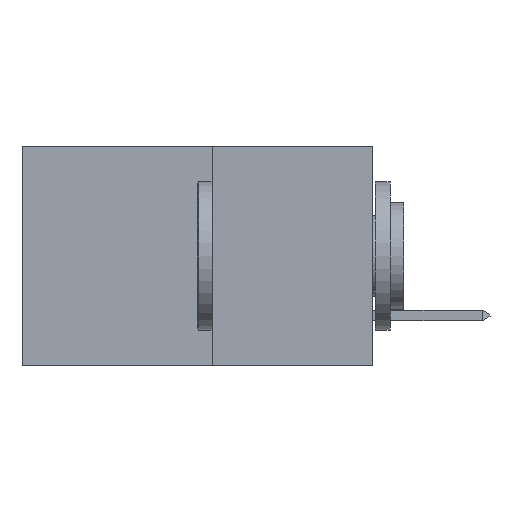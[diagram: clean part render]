
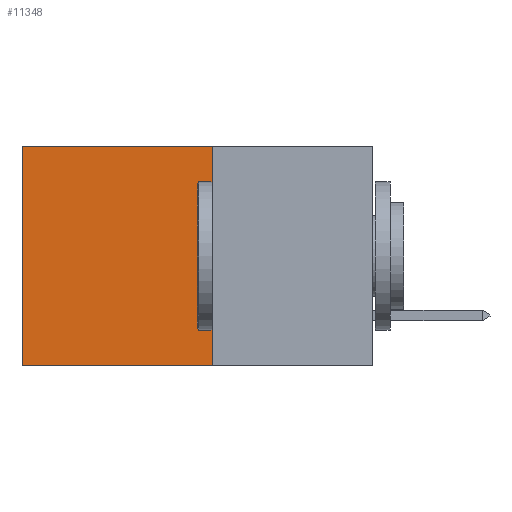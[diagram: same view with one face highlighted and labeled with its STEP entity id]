
A CAD part, left-side view. The second image highlights one B-rep face of the part: STEP entity #11348.
In plain terms, the highlighted planar face has unit normal (-1, 0, 0).
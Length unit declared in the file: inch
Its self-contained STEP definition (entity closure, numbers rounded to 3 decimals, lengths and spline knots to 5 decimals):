
#98 = FACE_OUTER_BOUND ( 'NONE', #2674, .T. ) ;
#156 = CARTESIAN_POINT ( 'NONE',  ( 0.277, 0.59, -0.37 ) ) ;
#1239 = ORIENTED_EDGE ( 'NONE', *, *, #2394, .F. ) ;
#1369 = VERTEX_POINT ( 'NONE', #7367 ) ;
#1559 = ORIENTED_EDGE ( 'NONE', *, *, #7161, .T. ) ;
#2394 = EDGE_CURVE ( 'NONE', #5105, #10106, #10455, .T. ) ;
#2674 = EDGE_LOOP ( 'NONE', ( #5955, #10576, #1239, #1559 ) ) ;
#2684 = DIRECTION ( 'NONE',  ( 0., 0., -1. ) ) ;
#2771 = CARTESIAN_POINT ( 'NONE',  ( 0.277, 0.59, 0. ) ) ;
#3268 = DIRECTION ( 'NONE',  ( 0., 0., -1. ) ) ;
#3438 = CARTESIAN_POINT ( 'NONE',  ( 0.277, 0.27, -0.37 ) ) ;
#3637 = VECTOR ( 'NONE', #2684, 39.37008 ) ;
#3905 = DIRECTION ( 'NONE',  ( 0., 1., 0. ) ) ;
#3999 = VECTOR ( 'NONE', #3905, 39.37008 ) ;
#4165 = LINE ( 'NONE', #156, #8921 ) ;
#4191 = AXIS2_PLACEMENT_3D ( 'NONE', #10374, #8700, #3268 ) ;
#4545 = LINE ( 'NONE', #6823, #8747 ) ;
#5105 = VERTEX_POINT ( 'NONE', #8084 ) ;
#5173 = CARTESIAN_POINT ( 'NONE',  ( 0.277, 0.27, -0.37 ) ) ;
#5481 = EDGE_CURVE ( 'NONE', #10106, #1369, #11046, .T. ) ;
#5955 = ORIENTED_EDGE ( 'NONE', *, *, #11228, .T. ) ;
#6306 = VERTEX_POINT ( 'NONE', #2771 ) ;
#6823 = CARTESIAN_POINT ( 'NONE',  ( 0.277, 0.27, 0. ) ) ;
#6907 = PLANE ( 'NONE',  #4191 ) ;
#7161 = EDGE_CURVE ( 'NONE', #5105, #6306, #4545, .T. ) ;
#7367 = CARTESIAN_POINT ( 'NONE',  ( 0.277, 0.59, -0.37 ) ) ;
#8084 = CARTESIAN_POINT ( 'NONE',  ( 0.277, 0.27, 0. ) ) ;
#8700 = DIRECTION ( 'NONE',  ( 1., 0., 0. ) ) ;
#8747 = VECTOR ( 'NONE', #11129, 39.37008 ) ;
#8921 = VECTOR ( 'NONE', #10190, 39.37008 ) ;
#10106 = VERTEX_POINT ( 'NONE', #11253 ) ;
#10190 = DIRECTION ( 'NONE',  ( 0., 0., -1. ) ) ;
#10374 = CARTESIAN_POINT ( 'NONE',  ( 0.277, 0.27, -0.37 ) ) ;
#10455 = LINE ( 'NONE', #3438, #3637 ) ;
#10576 = ORIENTED_EDGE ( 'NONE', *, *, #5481, .F. ) ;
#11046 = LINE ( 'NONE', #5173, #3999 ) ;
#11129 = DIRECTION ( 'NONE',  ( 0., 1., 0. ) ) ;
#11228 = EDGE_CURVE ( 'NONE', #6306, #1369, #4165, .T. ) ;
#11253 = CARTESIAN_POINT ( 'NONE',  ( 0.277, 0.27, -0.37 ) ) ;
#11348 = ADVANCED_FACE ( 'NONE', ( #98 ), #6907, .F. ) ;
